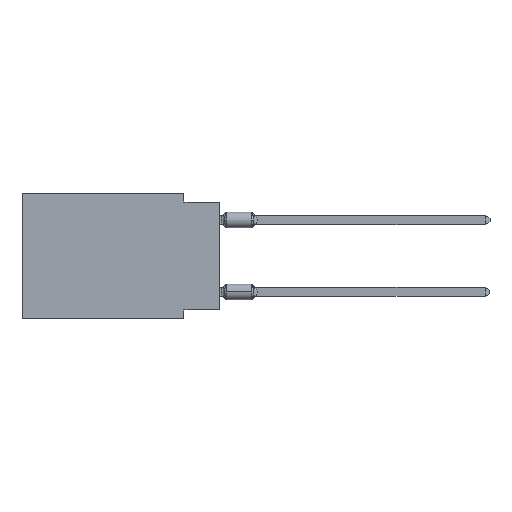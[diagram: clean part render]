
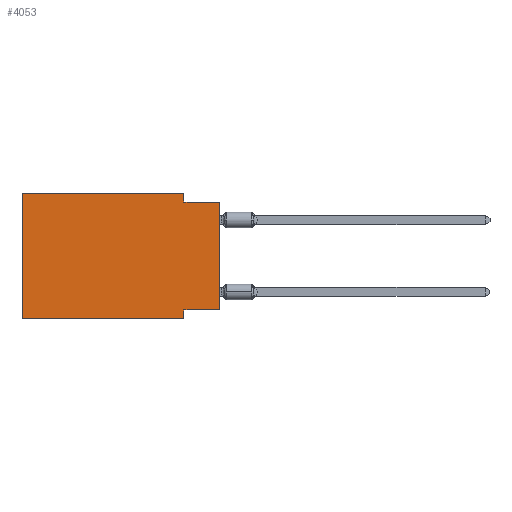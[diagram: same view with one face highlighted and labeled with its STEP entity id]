
A CAD part, left-side view. The second image highlights one B-rep face of the part: STEP entity #4053.
In plain terms, the highlighted planar face has unit normal (-1, 0, 0).
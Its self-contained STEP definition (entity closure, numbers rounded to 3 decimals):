
#11 = DIRECTION ( 'NONE',  ( 0., -1., 0. ) ) ;
#140 = LINE ( 'NONE', #9400, #9145 ) ;
#243 = VERTEX_POINT ( 'NONE', #3423 ) ;
#1292 = ORIENTED_EDGE ( 'NONE', *, *, #13713, .F. ) ;
#1753 = ORIENTED_EDGE ( 'NONE', *, *, #1850, .F. ) ;
#1850 = EDGE_CURVE ( 'NONE', #9056, #13568, #6324, .T. ) ;
#2191 = EDGE_CURVE ( 'NONE', #5825, #9056, #13498, .T. ) ;
#2511 = LINE ( 'NONE', #11776, #10192 ) ;
#2574 = EDGE_CURVE ( 'NONE', #10315, #5783, #13383, .T. ) ;
#2579 = EDGE_LOOP ( 'NONE', ( #14984, #13201, #7070, #1292, #7005, #4737, #1753, #4084 ) ) ;
#2880 = AXIS2_PLACEMENT_3D ( 'NONE', #6931, #5937, #9431 ) ;
#2909 = CARTESIAN_POINT ( 'NONE',  ( 0., 2.54, -0.635 ) ) ;
#2971 = CARTESIAN_POINT ( 'NONE',  ( 0., 0., -0.635 ) ) ;
#3052 = CARTESIAN_POINT ( 'NONE',  ( 0., 2.54, -8.255 ) ) ;
#3165 = CARTESIAN_POINT ( 'NONE',  ( 0., 13.97, 0. ) ) ;
#3230 = VECTOR ( 'NONE', #14429, 1000. ) ;
#3423 = CARTESIAN_POINT ( 'NONE',  ( 0., 13.97, -8.89 ) ) ;
#3432 = PLANE ( 'NONE',  #2880 ) ;
#3916 = EDGE_CURVE ( 'NONE', #7902, #10315, #12480, .T. ) ;
#4053 = ADVANCED_FACE ( 'NONE', ( #12637 ), #3432, .F. ) ;
#4084 = ORIENTED_EDGE ( 'NONE', *, *, #2191, .F. ) ;
#4364 = CARTESIAN_POINT ( 'NONE',  ( 0., 2.54, 0. ) ) ;
#4448 = VERTEX_POINT ( 'NONE', #6914 ) ;
#4632 = CARTESIAN_POINT ( 'NONE',  ( 0., 2.54, 0. ) ) ;
#4737 = ORIENTED_EDGE ( 'NONE', *, *, #10537, .T. ) ;
#4843 = VECTOR ( 'NONE', #6678, 1000. ) ;
#5013 = CARTESIAN_POINT ( 'NONE',  ( 0., 0., -8.255 ) ) ;
#5783 = VERTEX_POINT ( 'NONE', #13688 ) ;
#5825 = VERTEX_POINT ( 'NONE', #5013 ) ;
#5937 = DIRECTION ( 'NONE',  ( 1., 0., 0. ) ) ;
#6212 = VECTOR ( 'NONE', #10161, 1000. ) ;
#6324 = LINE ( 'NONE', #9799, #3230 ) ;
#6678 = DIRECTION ( 'NONE',  ( 0., 0., 1. ) ) ;
#6914 = CARTESIAN_POINT ( 'NONE',  ( 0., 13.97, 0. ) ) ;
#6931 = CARTESIAN_POINT ( 'NONE',  ( 0., 13.97, 0. ) ) ;
#7005 = ORIENTED_EDGE ( 'NONE', *, *, #12862, .F. ) ;
#7070 = ORIENTED_EDGE ( 'NONE', *, *, #3916, .F. ) ;
#7902 = VERTEX_POINT ( 'NONE', #4632 ) ;
#8713 = VECTOR ( 'NONE', #12408, 1000. ) ;
#8741 = LINE ( 'NONE', #11656, #4843 ) ;
#9056 = VERTEX_POINT ( 'NONE', #3052 ) ;
#9098 = LINE ( 'NONE', #3165, #6212 ) ;
#9145 = VECTOR ( 'NONE', #11, 1000. ) ;
#9400 = CARTESIAN_POINT ( 'NONE',  ( 0., 13.97, 0. ) ) ;
#9431 = DIRECTION ( 'NONE',  ( 0., 0., -1. ) ) ;
#9799 = CARTESIAN_POINT ( 'NONE',  ( 0., 2.54, -8.89 ) ) ;
#10161 = DIRECTION ( 'NONE',  ( 0., 0., 1. ) ) ;
#10192 = VECTOR ( 'NONE', #11700, 1000. ) ;
#10296 = VECTOR ( 'NONE', #12328, 1000. ) ;
#10315 = VERTEX_POINT ( 'NONE', #2909 ) ;
#10537 = EDGE_CURVE ( 'NONE', #243, #13568, #2511, .T. ) ;
#11148 = DIRECTION ( 'NONE',  ( 0., 1., 0. ) ) ;
#11181 = EDGE_CURVE ( 'NONE', #5825, #5783, #8741, .T. ) ;
#11656 = CARTESIAN_POINT ( 'NONE',  ( 0., 0., 0. ) ) ;
#11700 = DIRECTION ( 'NONE',  ( 0., -1., 0. ) ) ;
#11776 = CARTESIAN_POINT ( 'NONE',  ( 0., 13.97, -8.89 ) ) ;
#12228 = VECTOR ( 'NONE', #11148, 1000. ) ;
#12328 = DIRECTION ( 'NONE',  ( 0., -1., 0. ) ) ;
#12408 = DIRECTION ( 'NONE',  ( 0., 0., -1. ) ) ;
#12453 = CARTESIAN_POINT ( 'NONE',  ( 0., 2.54, -8.89 ) ) ;
#12480 = LINE ( 'NONE', #4364, #8713 ) ;
#12637 = FACE_OUTER_BOUND ( 'NONE', #2579, .T. ) ;
#12862 = EDGE_CURVE ( 'NONE', #243, #4448, #9098, .T. ) ;
#13201 = ORIENTED_EDGE ( 'NONE', *, *, #2574, .F. ) ;
#13354 = CARTESIAN_POINT ( 'NONE',  ( 0., 0., -8.255 ) ) ;
#13383 = LINE ( 'NONE', #2971, #10296 ) ;
#13498 = LINE ( 'NONE', #13354, #12228 ) ;
#13568 = VERTEX_POINT ( 'NONE', #12453 ) ;
#13688 = CARTESIAN_POINT ( 'NONE',  ( 0., 0., -0.635 ) ) ;
#13713 = EDGE_CURVE ( 'NONE', #4448, #7902, #140, .T. ) ;
#14429 = DIRECTION ( 'NONE',  ( 0., 0., -1. ) ) ;
#14984 = ORIENTED_EDGE ( 'NONE', *, *, #11181, .T. ) ;
